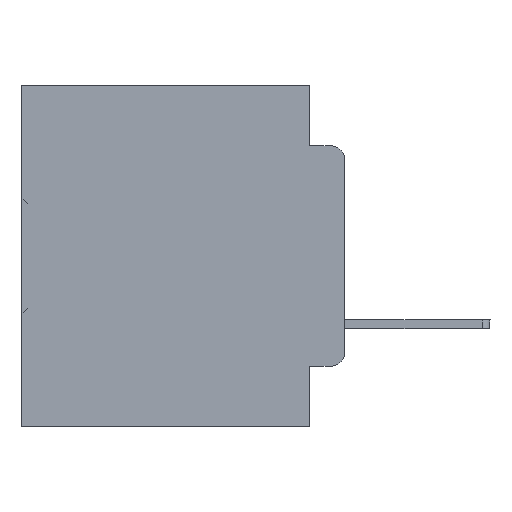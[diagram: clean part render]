
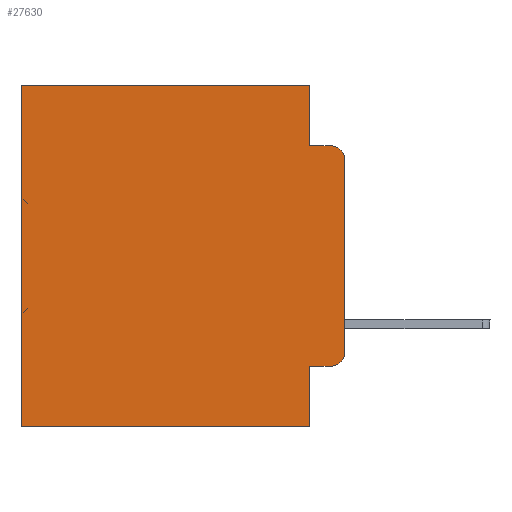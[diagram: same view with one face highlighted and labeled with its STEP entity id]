
A CAD part, left-side view. The second image highlights one B-rep face of the part: STEP entity #27630.
In plain terms, the highlighted planar face has unit normal (-1, 0, 0).
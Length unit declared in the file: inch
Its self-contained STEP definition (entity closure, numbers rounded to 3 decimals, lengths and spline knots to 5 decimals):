
#637 = CARTESIAN_POINT ( 'NONE',  ( 0.298, 0.02, -0.1085 ) ) ;
#697 = CARTESIAN_POINT ( 'NONE',  ( 0.298, 0.051, -0.5 ) ) ;
#831 = VERTEX_POINT ( 'NONE', #697 ) ;
#1168 = EDGE_CURVE ( 'NONE', #11796, #5993, #20214, .T. ) ;
#1173 = CARTESIAN_POINT ( 'NONE',  ( 0.298, 0.02, -0.3915 ) ) ;
#1227 = ORIENTED_EDGE ( 'NONE', *, *, #16240, .F. ) ;
#1482 = DIRECTION ( 'NONE',  ( 0., -1., 0. ) ) ;
#1884 = VECTOR ( 'NONE', #5507, 39.37008 ) ;
#1970 = ORIENTED_EDGE ( 'NONE', *, *, #6435, .T. ) ;
#2027 = LINE ( 'NONE', #22926, #35202 ) ;
#2096 = ORIENTED_EDGE ( 'NONE', *, *, #12496, .F. ) ;
#2651 = PLANE ( 'NONE',  #23234 ) ;
#3684 = CARTESIAN_POINT ( 'NONE',  ( 0.298, 0.02, -0.4115 ) ) ;
#4489 = CARTESIAN_POINT ( 'NONE',  ( 0.298, 0.051, -0.0885 ) ) ;
#4931 = ORIENTED_EDGE ( 'NONE', *, *, #1168, .T. ) ;
#5346 = VERTEX_POINT ( 'NONE', #25640 ) ;
#5507 = DIRECTION ( 'NONE',  ( 0., 0., -1. ) ) ;
#5657 = FACE_OUTER_BOUND ( 'NONE', #33641, .T. ) ;
#5993 = VERTEX_POINT ( 'NONE', #6956 ) ;
#6435 = EDGE_CURVE ( 'NONE', #16702, #26230, #16333, .T. ) ;
#6956 = CARTESIAN_POINT ( 'NONE',  ( 0.298, 0.473, 0. ) ) ;
#7772 = VECTOR ( 'NONE', #35098, 39.37008 ) ;
#7833 = ORIENTED_EDGE ( 'NONE', *, *, #22290, .T. ) ;
#8052 = CARTESIAN_POINT ( 'NONE',  ( 0.298, 0., -0.1085 ) ) ;
#8826 = ORIENTED_EDGE ( 'NONE', *, *, #15129, .T. ) ;
#9367 = DIRECTION ( 'NONE',  ( 0., 0., -1. ) ) ;
#10963 = CARTESIAN_POINT ( 'NONE',  ( 0.298, 0.051, -0.0885 ) ) ;
#11084 = VERTEX_POINT ( 'NONE', #8052 ) ;
#11129 = VECTOR ( 'NONE', #33001, 39.37008 ) ;
#11760 = DIRECTION ( 'NONE',  ( -1., 0., 0. ) ) ;
#11796 = VERTEX_POINT ( 'NONE', #24532 ) ;
#11909 = CARTESIAN_POINT ( 'NONE',  ( 0.298, 0.051, -0.4115 ) ) ;
#12183 = ORIENTED_EDGE ( 'NONE', *, *, #29781, .T. ) ;
#12452 = DIRECTION ( 'NONE',  ( 0., 0., -1. ) ) ;
#12496 = EDGE_CURVE ( 'NONE', #13876, #831, #19098, .T. ) ;
#13876 = VERTEX_POINT ( 'NONE', #11909 ) ;
#14704 = VECTOR ( 'NONE', #26792, 39.37008 ) ;
#14707 = CARTESIAN_POINT ( 'NONE',  ( 0.298, 0., -0.3915 ) ) ;
#15129 = EDGE_CURVE ( 'NONE', #5993, #5346, #16094, .T. ) ;
#15468 = LINE ( 'NONE', #33336, #11129 ) ;
#16094 = LINE ( 'NONE', #32276, #14704 ) ;
#16240 = EDGE_CURVE ( 'NONE', #34667, #18681, #33173, .T. ) ;
#16333 = CIRCLE ( 'NONE', #22262, 0.02 ) ;
#16702 = VERTEX_POINT ( 'NONE', #3684 ) ;
#18681 = VERTEX_POINT ( 'NONE', #19042 ) ;
#18832 = DIRECTION ( 'NONE',  ( 0., 0., -1. ) ) ;
#19042 = CARTESIAN_POINT ( 'NONE',  ( 0.298, 0.02, -0.0885 ) ) ;
#19098 = LINE ( 'NONE', #28874, #27603 ) ;
#19298 = DIRECTION ( 'NONE',  ( 1., 0., 0. ) ) ;
#19770 = EDGE_CURVE ( 'NONE', #11796, #34667, #25063, .T. ) ;
#20214 = LINE ( 'NONE', #26224, #7772 ) ;
#21321 = EDGE_CURVE ( 'NONE', #831, #5346, #23161, .T. ) ;
#21917 = CARTESIAN_POINT ( 'NONE',  ( 0.298, 0., 0. ) ) ;
#22262 = AXIS2_PLACEMENT_3D ( 'NONE', #1173, #31765, #31282 ) ;
#22290 = EDGE_CURVE ( 'NONE', #11084, #18681, #22597, .T. ) ;
#22335 = EDGE_CURVE ( 'NONE', #11084, #26230, #2027, .T. ) ;
#22597 = CIRCLE ( 'NONE', #26031, 0.02 ) ;
#22926 = CARTESIAN_POINT ( 'NONE',  ( 0.298, 0., 0. ) ) ;
#23161 = LINE ( 'NONE', #25863, #29649 ) ;
#23234 = AXIS2_PLACEMENT_3D ( 'NONE', #21917, #19298, #18832 ) ;
#23381 = ORIENTED_EDGE ( 'NONE', *, *, #22335, .F. ) ;
#24532 = CARTESIAN_POINT ( 'NONE',  ( 0.298, 0.051, 0. ) ) ;
#25063 = LINE ( 'NONE', #32132, #1884 ) ;
#25070 = ORIENTED_EDGE ( 'NONE', *, *, #19770, .F. ) ;
#25336 = VECTOR ( 'NONE', #1482, 39.37008 ) ;
#25640 = CARTESIAN_POINT ( 'NONE',  ( 0.298, 0.473, -0.5 ) ) ;
#25863 = CARTESIAN_POINT ( 'NONE',  ( 0.298, 0., -0.5 ) ) ;
#26031 = AXIS2_PLACEMENT_3D ( 'NONE', #637, #11760, #28308 ) ;
#26224 = CARTESIAN_POINT ( 'NONE',  ( 0.298, 0., 0. ) ) ;
#26230 = VERTEX_POINT ( 'NONE', #14707 ) ;
#26792 = DIRECTION ( 'NONE',  ( 0., 0., -1. ) ) ;
#27603 = VECTOR ( 'NONE', #12452, 39.37008 ) ;
#27630 = ADVANCED_FACE ( 'NONE', ( #5657 ), #2651, .F. ) ;
#28308 = DIRECTION ( 'NONE',  ( 0., 0., -1. ) ) ;
#28874 = CARTESIAN_POINT ( 'NONE',  ( 0.298, 0.051, 0. ) ) ;
#29649 = VECTOR ( 'NONE', #34093, 39.37008 ) ;
#29781 = EDGE_CURVE ( 'NONE', #13876, #16702, #15468, .T. ) ;
#31282 = DIRECTION ( 'NONE',  ( 0., 0., -1. ) ) ;
#31765 = DIRECTION ( 'NONE',  ( -1., 0., 0. ) ) ;
#32132 = CARTESIAN_POINT ( 'NONE',  ( 0.298, 0.051, 0. ) ) ;
#32276 = CARTESIAN_POINT ( 'NONE',  ( 0.298, 0.473, 0. ) ) ;
#32670 = ORIENTED_EDGE ( 'NONE', *, *, #21321, .F. ) ;
#33001 = DIRECTION ( 'NONE',  ( 0., -1., 0. ) ) ;
#33173 = LINE ( 'NONE', #4489, #25336 ) ;
#33336 = CARTESIAN_POINT ( 'NONE',  ( 0.298, 0.051, -0.4115 ) ) ;
#33641 = EDGE_LOOP ( 'NONE', ( #23381, #7833, #1227, #25070, #4931, #8826, #32670, #2096, #12183, #1970 ) ) ;
#34093 = DIRECTION ( 'NONE',  ( 0., 1., 0. ) ) ;
#34667 = VERTEX_POINT ( 'NONE', #10963 ) ;
#35098 = DIRECTION ( 'NONE',  ( 0., 1., 0. ) ) ;
#35202 = VECTOR ( 'NONE', #9367, 39.37008 ) ;
